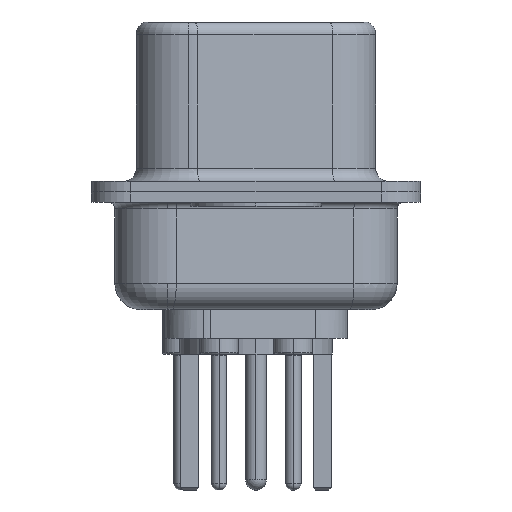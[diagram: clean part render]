
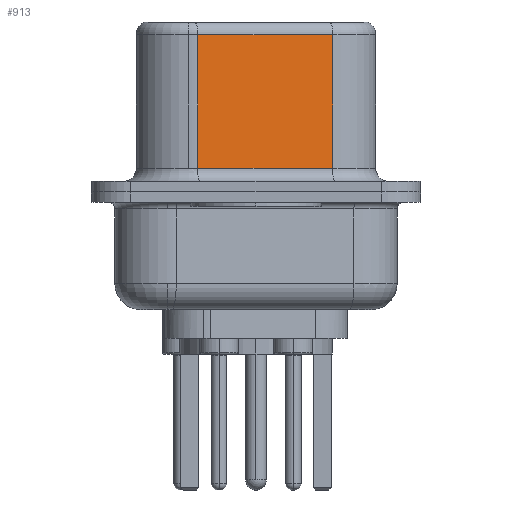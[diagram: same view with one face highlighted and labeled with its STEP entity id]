
A CAD part, left-side view. The second image highlights one B-rep face of the part: STEP entity #913.
In plain terms, the highlighted planar face has unit normal (-0.985, -0.174, 0).
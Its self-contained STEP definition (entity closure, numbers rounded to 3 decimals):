
#913 = ADVANCED_FACE ( 'NONE', ( #8999 ), #14239, .F. ) ;
#3003 = LINE ( 'NONE', #11850, #19966 ) ;
#3037 = VERTEX_POINT ( 'NONE', #5450 ) ;
#3313 = CARTESIAN_POINT ( 'NONE',  ( 4.585, -2.927, 6.52 ) ) ;
#3487 = VERTEX_POINT ( 'NONE', #9946 ) ;
#3563 = LINE ( 'NONE', #12738, #18524 ) ;
#3684 = LINE ( 'NONE', #20346, #17352 ) ;
#5450 = CARTESIAN_POINT ( 'NONE',  ( 3.675, 2.233, 6.02 ) ) ;
#5567 = DIRECTION ( 'NONE',  ( 0.174, -0.985, 0. ) ) ;
#6230 = EDGE_CURVE ( 'NONE', #21186, #3037, #3003, .T. ) ;
#6457 = CARTESIAN_POINT ( 'NONE',  ( 4.585, -2.927, 0.9 ) ) ;
#7664 = CARTESIAN_POINT ( 'NONE',  ( 4.585, -2.927, 6.52 ) ) ;
#7835 = DIRECTION ( 'NONE',  ( 0., 0., -1. ) ) ;
#8487 = EDGE_CURVE ( 'NONE', #3487, #16706, #3684, .T. ) ;
#8999 = FACE_OUTER_BOUND ( 'NONE', #11732, .T. ) ;
#9326 = DIRECTION ( 'NONE',  ( 0.985, 0.174, 0. ) ) ;
#9327 = ORIENTED_EDGE ( 'NONE', *, *, #6230, .T. ) ;
#9891 = ORIENTED_EDGE ( 'NONE', *, *, #8487, .T. ) ;
#9946 = CARTESIAN_POINT ( 'NONE',  ( 3.675, 2.233, 0.9 ) ) ;
#11732 = EDGE_LOOP ( 'NONE', ( #19676, #9327, #15817, #9891 ) ) ;
#11850 = CARTESIAN_POINT ( 'NONE',  ( 4.585, -2.927, 6.02 ) ) ;
#12506 = DIRECTION ( 'NONE',  ( 0., 0., -1. ) ) ;
#12738 = CARTESIAN_POINT ( 'NONE',  ( 3.675, 2.233, 6.52 ) ) ;
#14239 = PLANE ( 'NONE',  #16050 ) ;
#14621 = CARTESIAN_POINT ( 'NONE',  ( 4.585, -2.927, 6.02 ) ) ;
#14632 = LINE ( 'NONE', #3313, #19224 ) ;
#15628 = DIRECTION ( 'NONE',  ( -0.174, 0.985, 0. ) ) ;
#15817 = ORIENTED_EDGE ( 'NONE', *, *, #16874, .T. ) ;
#16050 = AXIS2_PLACEMENT_3D ( 'NONE', #7664, #9326, #15628 ) ;
#16706 = VERTEX_POINT ( 'NONE', #6457 ) ;
#16858 = DIRECTION ( 'NONE',  ( -0.174, 0.985, 0. ) ) ;
#16874 = EDGE_CURVE ( 'NONE', #3037, #3487, #3563, .T. ) ;
#17352 = VECTOR ( 'NONE', #5567, 1000. ) ;
#18524 = VECTOR ( 'NONE', #7835, 1000. ) ;
#19224 = VECTOR ( 'NONE', #12506, 1000. ) ;
#19676 = ORIENTED_EDGE ( 'NONE', *, *, #20050, .F. ) ;
#19966 = VECTOR ( 'NONE', #16858, 1000. ) ;
#20050 = EDGE_CURVE ( 'NONE', #21186, #16706, #14632, .T. ) ;
#20346 = CARTESIAN_POINT ( 'NONE',  ( 4.585, -2.927, 0.9 ) ) ;
#21186 = VERTEX_POINT ( 'NONE', #14621 ) ;
